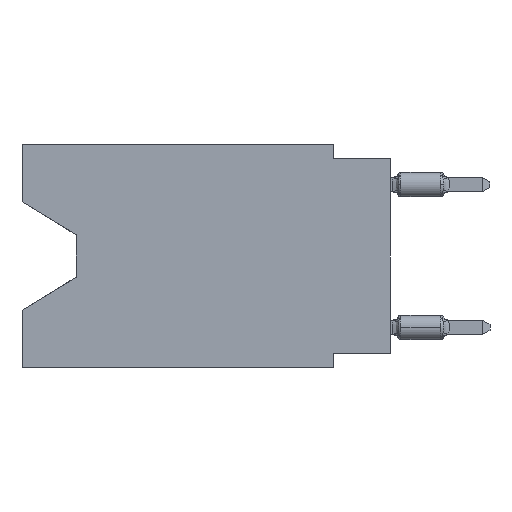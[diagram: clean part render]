
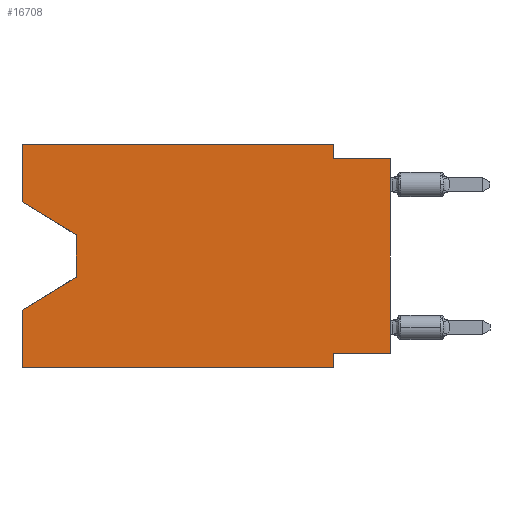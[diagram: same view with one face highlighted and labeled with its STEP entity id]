
A CAD part, left-side view. The second image highlights one B-rep face of the part: STEP entity #16708.
In plain terms, the highlighted planar face has unit normal (-1, 0, 0).
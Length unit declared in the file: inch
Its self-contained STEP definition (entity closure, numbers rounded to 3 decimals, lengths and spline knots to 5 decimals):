
#76 = CARTESIAN_POINT ( 'NONE',  ( 0., 0., -0.025 ) ) ;
#145 = VERTEX_POINT ( 'NONE', #5476 ) ;
#224 = DIRECTION ( 'NONE',  ( 0., 0., -1. ) ) ;
#431 = VECTOR ( 'NONE', #10906, 39.37008 ) ;
#648 = VECTOR ( 'NONE', #4388, 39.37008 ) ;
#718 = DIRECTION ( 'NONE',  ( 1., 0., 0. ) ) ;
#827 = PLANE ( 'NONE',  #3398 ) ;
#838 = CARTESIAN_POINT ( 'NONE',  ( 0., 0.645, 0. ) ) ;
#944 = CARTESIAN_POINT ( 'NONE',  ( 0., 0.645, -0.10025 ) ) ;
#1628 = CARTESIAN_POINT ( 'NONE',  ( 0., 0.645, -0.28975 ) ) ;
#1638 = CARTESIAN_POINT ( 'NONE',  ( 0., 0.645, -0.10025 ) ) ;
#2187 = VECTOR ( 'NONE', #12242, 39.37008 ) ;
#2350 = FACE_OUTER_BOUND ( 'NONE', #17371, .T. ) ;
#2454 = ORIENTED_EDGE ( 'NONE', *, *, #16655, .F. ) ;
#2467 = DIRECTION ( 'NONE',  ( 0., 0., 1. ) ) ;
#2475 = CARTESIAN_POINT ( 'NONE',  ( 0., 0.1, 0. ) ) ;
#2579 = LINE ( 'NONE', #2881, #2187 ) ;
#2618 = ORIENTED_EDGE ( 'NONE', *, *, #10043, .T. ) ;
#2817 = DIRECTION ( 'NONE',  ( 0., 1., 0. ) ) ;
#2881 = CARTESIAN_POINT ( 'NONE',  ( 0., 0.1, -0.39 ) ) ;
#3187 = EDGE_CURVE ( 'NONE', #17890, #4445, #13159, .T. ) ;
#3386 = CARTESIAN_POINT ( 'NONE',  ( 0., 0.1, -0.365 ) ) ;
#3398 = AXIS2_PLACEMENT_3D ( 'NONE', #19502, #718, #11918 ) ;
#3642 = VERTEX_POINT ( 'NONE', #17112 ) ;
#3828 = LINE ( 'NONE', #19658, #11842 ) ;
#4101 = VERTEX_POINT ( 'NONE', #3386 ) ;
#4150 = VECTOR ( 'NONE', #5833, 39.37008 ) ;
#4159 = VERTEX_POINT ( 'NONE', #15832 ) ;
#4238 = CARTESIAN_POINT ( 'NONE',  ( 0., 0., -0.365 ) ) ;
#4388 = DIRECTION ( 'NONE',  ( 0., 0., 1. ) ) ;
#4445 = VERTEX_POINT ( 'NONE', #1628 ) ;
#4780 = ORIENTED_EDGE ( 'NONE', *, *, #5945, .F. ) ;
#4938 = VECTOR ( 'NONE', #2467, 39.37008 ) ;
#5223 = ORIENTED_EDGE ( 'NONE', *, *, #9648, .F. ) ;
#5413 = CARTESIAN_POINT ( 'NONE',  ( 0., 0.1, -0.39 ) ) ;
#5416 = VERTEX_POINT ( 'NONE', #5413 ) ;
#5476 = CARTESIAN_POINT ( 'NONE',  ( 0., 0.645, 0. ) ) ;
#5592 = CARTESIAN_POINT ( 'NONE',  ( 0., 0.1, -0.025 ) ) ;
#5739 = CARTESIAN_POINT ( 'NONE',  ( 0., 0.645, -0.39 ) ) ;
#5813 = LINE ( 'NONE', #8880, #648 ) ;
#5833 = DIRECTION ( 'NONE',  ( 0., -1., 0. ) ) ;
#5912 = VERTEX_POINT ( 'NONE', #4238 ) ;
#5945 = EDGE_CURVE ( 'NONE', #5912, #4101, #10550, .T. ) ;
#6225 = VERTEX_POINT ( 'NONE', #944 ) ;
#6327 = LINE ( 'NONE', #1638, #431 ) ;
#6739 = ORIENTED_EDGE ( 'NONE', *, *, #11808, .F. ) ;
#7565 = DIRECTION ( 'NONE',  ( 0., 0., -1. ) ) ;
#7643 = ORIENTED_EDGE ( 'NONE', *, *, #15001, .T. ) ;
#7673 = CARTESIAN_POINT ( 'NONE',  ( 0., 0.55, -0.158 ) ) ;
#7966 = CARTESIAN_POINT ( 'NONE',  ( 0., 0.1, 0. ) ) ;
#8184 = ORIENTED_EDGE ( 'NONE', *, *, #17581, .F. ) ;
#8595 = CARTESIAN_POINT ( 'NONE',  ( 0., 0.645, -0.39 ) ) ;
#8880 = CARTESIAN_POINT ( 'NONE',  ( 0., 0., 0. ) ) ;
#9308 = VERTEX_POINT ( 'NONE', #5592 ) ;
#9512 = VECTOR ( 'NONE', #2817, 39.37008 ) ;
#9644 = EDGE_CURVE ( 'NONE', #17890, #5416, #13482, .T. ) ;
#9648 = EDGE_CURVE ( 'NONE', #4101, #5416, #2579, .T. ) ;
#9901 = CARTESIAN_POINT ( 'NONE',  ( 0., 0.55, -0.232 ) ) ;
#10043 = EDGE_CURVE ( 'NONE', #5912, #4159, #5813, .T. ) ;
#10155 = CARTESIAN_POINT ( 'NONE',  ( 0., 0., -0.365 ) ) ;
#10470 = VECTOR ( 'NONE', #15778, 39.37008 ) ;
#10550 = LINE ( 'NONE', #10155, #9512 ) ;
#10906 = DIRECTION ( 'NONE',  ( 0., -0.855, -0.519 ) ) ;
#10907 = ORIENTED_EDGE ( 'NONE', *, *, #3187, .F. ) ;
#11308 = LINE ( 'NONE', #7966, #15784 ) ;
#11808 = EDGE_CURVE ( 'NONE', #9308, #4159, #18554, .T. ) ;
#11842 = VECTOR ( 'NONE', #18119, 39.37008 ) ;
#11918 = DIRECTION ( 'NONE',  ( 0., 0., -1. ) ) ;
#11940 = CARTESIAN_POINT ( 'NONE',  ( 0., 0.55, -0.232 ) ) ;
#12131 = VECTOR ( 'NONE', #18795, 39.37008 ) ;
#12242 = DIRECTION ( 'NONE',  ( 0., 0., -1. ) ) ;
#12638 = ORIENTED_EDGE ( 'NONE', *, *, #15023, .T. ) ;
#12999 = LINE ( 'NONE', #13958, #20082 ) ;
#13159 = LINE ( 'NONE', #838, #4938 ) ;
#13482 = LINE ( 'NONE', #5739, #4150 ) ;
#13578 = VERTEX_POINT ( 'NONE', #2475 ) ;
#13673 = EDGE_CURVE ( 'NONE', #3642, #19578, #16755, .T. ) ;
#13893 = ORIENTED_EDGE ( 'NONE', *, *, #13673, .T. ) ;
#13958 = CARTESIAN_POINT ( 'NONE',  ( 0., 0.645, 0. ) ) ;
#13972 = LINE ( 'NONE', #11940, #12131 ) ;
#15001 = EDGE_CURVE ( 'NONE', #19578, #4445, #13972, .T. ) ;
#15023 = EDGE_CURVE ( 'NONE', #6225, #3642, #6327, .T. ) ;
#15699 = VECTOR ( 'NONE', #7565, 39.37008 ) ;
#15778 = DIRECTION ( 'NONE',  ( 0., -1., 0. ) ) ;
#15784 = VECTOR ( 'NONE', #224, 39.37008 ) ;
#15832 = CARTESIAN_POINT ( 'NONE',  ( 0., 0., -0.025 ) ) ;
#16655 = EDGE_CURVE ( 'NONE', #13578, #9308, #11308, .T. ) ;
#16708 = ADVANCED_FACE ( 'NONE', ( #2350 ), #827, .F. ) ;
#16755 = LINE ( 'NONE', #7673, #15699 ) ;
#17112 = CARTESIAN_POINT ( 'NONE',  ( 0., 0.55, -0.158 ) ) ;
#17136 = DIRECTION ( 'NONE',  ( 0., 0., 1. ) ) ;
#17371 = EDGE_LOOP ( 'NONE', ( #12638, #13893, #7643, #10907, #20181, #5223, #4780, #2618, #6739, #2454, #8184, #17569 ) ) ;
#17569 = ORIENTED_EDGE ( 'NONE', *, *, #19845, .F. ) ;
#17581 = EDGE_CURVE ( 'NONE', #145, #13578, #3828, .T. ) ;
#17890 = VERTEX_POINT ( 'NONE', #8595 ) ;
#18119 = DIRECTION ( 'NONE',  ( 0., -1., 0. ) ) ;
#18554 = LINE ( 'NONE', #76, #10470 ) ;
#18795 = DIRECTION ( 'NONE',  ( 0., 0.855, -0.519 ) ) ;
#19502 = CARTESIAN_POINT ( 'NONE',  ( 0., 0.645, 0. ) ) ;
#19578 = VERTEX_POINT ( 'NONE', #9901 ) ;
#19658 = CARTESIAN_POINT ( 'NONE',  ( 0., 0.645, 0. ) ) ;
#19845 = EDGE_CURVE ( 'NONE', #6225, #145, #12999, .T. ) ;
#20082 = VECTOR ( 'NONE', #17136, 39.37008 ) ;
#20181 = ORIENTED_EDGE ( 'NONE', *, *, #9644, .T. ) ;
